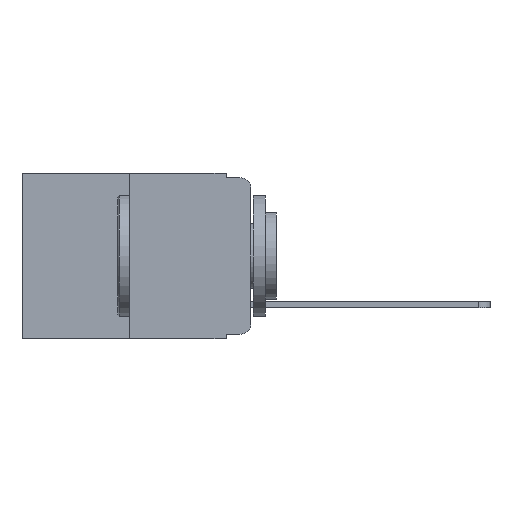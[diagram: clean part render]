
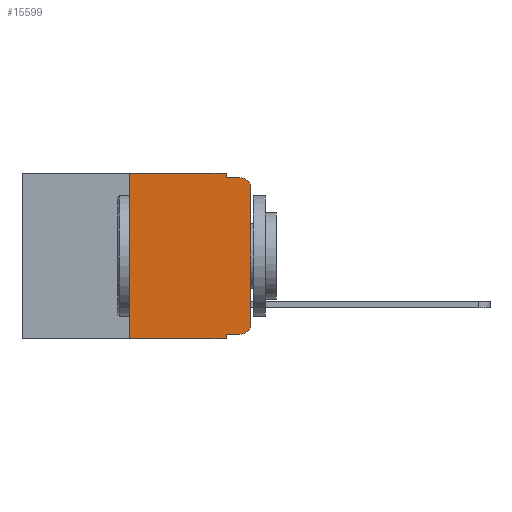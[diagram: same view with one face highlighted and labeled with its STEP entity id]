
A CAD part, left-side view. The second image highlights one B-rep face of the part: STEP entity #15599.
In plain terms, the highlighted planar face has unit normal (-1, 0, 0).
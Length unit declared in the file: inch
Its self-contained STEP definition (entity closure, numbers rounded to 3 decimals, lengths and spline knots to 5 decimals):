
#313 = ORIENTED_EDGE ( 'NONE', *, *, #21103, .T. ) ;
#363 = LINE ( 'NONE', #1667, #14607 ) ;
#477 = VERTEX_POINT ( 'NONE', #1755 ) ;
#797 = CARTESIAN_POINT ( 'NONE',  ( 0., 0.051, 0. ) ) ;
#1089 = CIRCLE ( 'NONE', #3849, 0.02 ) ;
#1129 = CARTESIAN_POINT ( 'NONE',  ( 0., 0.02, -0.313 ) ) ;
#1634 = VERTEX_POINT ( 'NONE', #13103 ) ;
#1667 = CARTESIAN_POINT ( 'NONE',  ( 0., 0.473, -0.343 ) ) ;
#1755 = CARTESIAN_POINT ( 'NONE',  ( 0., 0., -0.03 ) ) ;
#1819 = DIRECTION ( 'NONE',  ( -1., 0., 0. ) ) ;
#2250 = CARTESIAN_POINT ( 'NONE',  ( 0., 0.051, -0.01 ) ) ;
#2363 = DIRECTION ( 'NONE',  ( 0., -1., 0. ) ) ;
#2505 = CARTESIAN_POINT ( 'NONE',  ( 0., 0.02, -0.333 ) ) ;
#2522 = ORIENTED_EDGE ( 'NONE', *, *, #6725, .F. ) ;
#2623 = DIRECTION ( 'NONE',  ( 0., 0., -1. ) ) ;
#2831 = AXIS2_PLACEMENT_3D ( 'NONE', #21275, #15703, #4358 ) ;
#3047 = DIRECTION ( 'NONE',  ( 0., -1., 0. ) ) ;
#3849 = AXIS2_PLACEMENT_3D ( 'NONE', #1129, #12363, #6998 ) ;
#4358 = DIRECTION ( 'NONE',  ( 0., 0., -1. ) ) ;
#4600 = EDGE_CURVE ( 'NONE', #477, #23336, #16914, .T. ) ;
#4714 = CARTESIAN_POINT ( 'NONE',  ( 0., 0.051, -0.333 ) ) ;
#4762 = VECTOR ( 'NONE', #2363, 39.37008 ) ;
#5443 = VERTEX_POINT ( 'NONE', #16866 ) ;
#5739 = EDGE_LOOP ( 'NONE', ( #313, #21388, #16619, #10198, #21635, #2522, #21334, #23279, #23434, #22123 ) ) ;
#5924 = CARTESIAN_POINT ( 'NONE',  ( 0., 0.051, -0.333 ) ) ;
#6053 = DIRECTION ( 'NONE',  ( 0., -1., 0. ) ) ;
#6380 = DIRECTION ( 'NONE',  ( 0., 0., 1. ) ) ;
#6725 = EDGE_CURVE ( 'NONE', #16937, #1634, #13074, .T. ) ;
#6998 = DIRECTION ( 'NONE',  ( 0., 0., -1. ) ) ;
#7974 = CARTESIAN_POINT ( 'NONE',  ( 0., 0.051, -0.343 ) ) ;
#8885 = VERTEX_POINT ( 'NONE', #2505 ) ;
#9102 = VECTOR ( 'NONE', #2623, 39.37008 ) ;
#9166 = EDGE_CURVE ( 'NONE', #16282, #22718, #21300, .T. ) ;
#10035 = EDGE_CURVE ( 'NONE', #8885, #20408, #1089, .T. ) ;
#10198 = ORIENTED_EDGE ( 'NONE', *, *, #18771, .F. ) ;
#10768 = FACE_OUTER_BOUND ( 'NONE', #5739, .T. ) ;
#10884 = VERTEX_POINT ( 'NONE', #13168 ) ;
#11070 = VECTOR ( 'NONE', #20944, 39.37008 ) ;
#11600 = CARTESIAN_POINT ( 'NONE',  ( 0., 0., 0. ) ) ;
#12135 = LINE ( 'NONE', #11600, #12751 ) ;
#12363 = DIRECTION ( 'NONE',  ( -1., 0., 0. ) ) ;
#12751 = VECTOR ( 'NONE', #13262, 39.37008 ) ;
#13074 = LINE ( 'NONE', #13750, #14563 ) ;
#13103 = CARTESIAN_POINT ( 'NONE',  ( 0., 0.25, 0. ) ) ;
#13168 = CARTESIAN_POINT ( 'NONE',  ( 0., 0.051, -0.01 ) ) ;
#13262 = DIRECTION ( 'NONE',  ( 0., 0., 1. ) ) ;
#13541 = LINE ( 'NONE', #2250, #23662 ) ;
#13750 = CARTESIAN_POINT ( 'NONE',  ( 0., 0.25, 0. ) ) ;
#13812 = CARTESIAN_POINT ( 'NONE',  ( 0., 0.02, -0.01 ) ) ;
#14030 = PLANE ( 'NONE',  #2831 ) ;
#14563 = VECTOR ( 'NONE', #6380, 39.37008 ) ;
#14607 = VECTOR ( 'NONE', #24315, 39.37008 ) ;
#15599 = ADVANCED_FACE ( 'NONE', ( #10768 ), #14030, .F. ) ;
#15703 = DIRECTION ( 'NONE',  ( 1., 0., 0. ) ) ;
#16282 = VERTEX_POINT ( 'NONE', #4714 ) ;
#16619 = ORIENTED_EDGE ( 'NONE', *, *, #23408, .F. ) ;
#16866 = CARTESIAN_POINT ( 'NONE',  ( 0., 0.051, 0. ) ) ;
#16914 = CIRCLE ( 'NONE', #22177, 0.02 ) ;
#16937 = VERTEX_POINT ( 'NONE', #18115 ) ;
#17372 = VECTOR ( 'NONE', #3047, 39.37008 ) ;
#18115 = CARTESIAN_POINT ( 'NONE',  ( 0., 0.25, -0.343 ) ) ;
#18600 = LINE ( 'NONE', #23812, #17372 ) ;
#18771 = EDGE_CURVE ( 'NONE', #5443, #10884, #20306, .T. ) ;
#18948 = CARTESIAN_POINT ( 'NONE',  ( 0., 0., -0.313 ) ) ;
#19023 = CARTESIAN_POINT ( 'NONE',  ( 0., 0.051, 0. ) ) ;
#19186 = EDGE_CURVE ( 'NONE', #16937, #22718, #363, .T. ) ;
#20306 = LINE ( 'NONE', #19023, #11070 ) ;
#20408 = VERTEX_POINT ( 'NONE', #18948 ) ;
#20602 = EDGE_CURVE ( 'NONE', #16282, #8885, #21371, .T. ) ;
#20906 = DIRECTION ( 'NONE',  ( 0., 0., -1. ) ) ;
#20944 = DIRECTION ( 'NONE',  ( 0., 0., -1. ) ) ;
#21103 = EDGE_CURVE ( 'NONE', #20408, #477, #12135, .T. ) ;
#21275 = CARTESIAN_POINT ( 'NONE',  ( 0., 0.473, 0. ) ) ;
#21300 = LINE ( 'NONE', #797, #9102 ) ;
#21334 = ORIENTED_EDGE ( 'NONE', *, *, #19186, .T. ) ;
#21371 = LINE ( 'NONE', #5924, #4762 ) ;
#21388 = ORIENTED_EDGE ( 'NONE', *, *, #4600, .T. ) ;
#21635 = ORIENTED_EDGE ( 'NONE', *, *, #22951, .F. ) ;
#22123 = ORIENTED_EDGE ( 'NONE', *, *, #10035, .T. ) ;
#22177 = AXIS2_PLACEMENT_3D ( 'NONE', #24541, #1819, #20906 ) ;
#22718 = VERTEX_POINT ( 'NONE', #7974 ) ;
#22951 = EDGE_CURVE ( 'NONE', #1634, #5443, #18600, .T. ) ;
#23279 = ORIENTED_EDGE ( 'NONE', *, *, #9166, .F. ) ;
#23336 = VERTEX_POINT ( 'NONE', #13812 ) ;
#23408 = EDGE_CURVE ( 'NONE', #10884, #23336, #13541, .T. ) ;
#23434 = ORIENTED_EDGE ( 'NONE', *, *, #20602, .T. ) ;
#23662 = VECTOR ( 'NONE', #6053, 39.37008 ) ;
#23812 = CARTESIAN_POINT ( 'NONE',  ( 0., 0.473, 0. ) ) ;
#24315 = DIRECTION ( 'NONE',  ( 0., -1., 0. ) ) ;
#24541 = CARTESIAN_POINT ( 'NONE',  ( 0., 0.02, -0.03 ) ) ;
